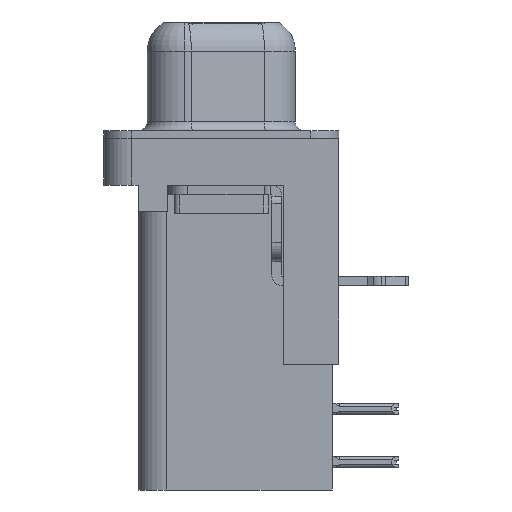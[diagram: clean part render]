
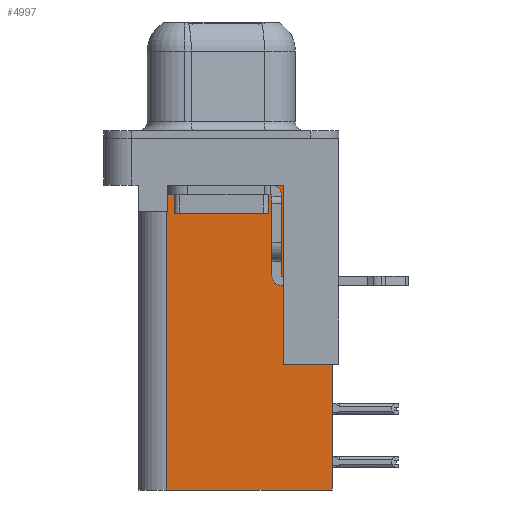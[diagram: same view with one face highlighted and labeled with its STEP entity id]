
A CAD part, left-side view. The second image highlights one B-rep face of the part: STEP entity #4997.
In plain terms, the highlighted planar face has unit normal (-1, 0, 0).
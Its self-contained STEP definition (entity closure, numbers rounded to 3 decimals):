
#1304 = CARTESIAN_POINT ( 'NONE',  ( 3.79, 2.925, -3.9 ) ) ;
#1524 = LINE ( 'NONE', #13325, #19295 ) ;
#1573 = ORIENTED_EDGE ( 'NONE', *, *, #17814, .F. ) ;
#1762 = LINE ( 'NONE', #19416, #5287 ) ;
#1792 = CARTESIAN_POINT ( 'NONE',  ( 3.79, -3.295, -12.05 ) ) ;
#2110 = CARTESIAN_POINT ( 'NONE',  ( 3.79, -3.295, -18.76 ) ) ;
#2253 = DIRECTION ( 'NONE',  ( 0., 0., -1. ) ) ;
#2333 = CARTESIAN_POINT ( 'NONE',  ( 3.79, 2.895, -2.5 ) ) ;
#2478 = CARTESIAN_POINT ( 'NONE',  ( 3.79, 2.925, -18.76 ) ) ;
#2762 = VERTEX_POINT ( 'NONE', #1304 ) ;
#3011 = VECTOR ( 'NONE', #16587, 1000. ) ;
#3033 = DIRECTION ( 'NONE',  ( 0., 1., 0. ) ) ;
#3044 = ORIENTED_EDGE ( 'NONE', *, *, #13088, .T. ) ;
#4007 = CARTESIAN_POINT ( 'NONE',  ( 3.79, 2.925, -18.76 ) ) ;
#4114 = ORIENTED_EDGE ( 'NONE', *, *, #16020, .T. ) ;
#4213 = ORIENTED_EDGE ( 'NONE', *, *, #9682, .F. ) ;
#4594 = CARTESIAN_POINT ( 'NONE',  ( 3.79, -5.925, -2. ) ) ;
#4817 = EDGE_CURVE ( 'NONE', #7934, #2762, #17651, .T. ) ;
#4990 = DIRECTION ( 'NONE',  ( 0., 0., 1. ) ) ;
#4997 = ADVANCED_FACE ( 'NONE', ( #9859 ), #18794, .F. ) ;
#5287 = VECTOR ( 'NONE', #21104, 1000. ) ;
#5357 = CARTESIAN_POINT ( 'NONE',  ( 3.79, -3.295, -18.76 ) ) ;
#5561 = VECTOR ( 'NONE', #8408, 1000. ) ;
#5635 = ORIENTED_EDGE ( 'NONE', *, *, #21165, .T. ) ;
#7562 = EDGE_LOOP ( 'NONE', ( #5635, #3044, #20001, #19280, #1573, #4213, #4114, #18623 ) ) ;
#7934 = VERTEX_POINT ( 'NONE', #2478 ) ;
#8408 = DIRECTION ( 'NONE',  ( 0., 1., 0. ) ) ;
#8547 = VERTEX_POINT ( 'NONE', #11242 ) ;
#9682 = EDGE_CURVE ( 'NONE', #17001, #17704, #16182, .T. ) ;
#9859 = FACE_OUTER_BOUND ( 'NONE', #7562, .T. ) ;
#10117 = CARTESIAN_POINT ( 'NONE',  ( 3.79, 0., -3.9 ) ) ;
#10385 = VECTOR ( 'NONE', #20947, 1000. ) ;
#10558 = CARTESIAN_POINT ( 'NONE',  ( 3.79, -5.925, -18.76 ) ) ;
#10758 = VERTEX_POINT ( 'NONE', #2333 ) ;
#10922 = LINE ( 'NONE', #2110, #10385 ) ;
#11242 = CARTESIAN_POINT ( 'NONE',  ( 3.79, -3.295, -2.5 ) ) ;
#11509 = LINE ( 'NONE', #12554, #20598 ) ;
#12386 = VERTEX_POINT ( 'NONE', #16503 ) ;
#12554 = CARTESIAN_POINT ( 'NONE',  ( 3.79, 2.895, -3.9 ) ) ;
#12839 = AXIS2_PLACEMENT_3D ( 'NONE', #5357, #17766, #17735 ) ;
#13088 = EDGE_CURVE ( 'NONE', #10758, #12386, #11509, .T. ) ;
#13325 = CARTESIAN_POINT ( 'NONE',  ( 3.79, -6.295, -12.05 ) ) ;
#14022 = EDGE_CURVE ( 'NONE', #12386, #2762, #19263, .T. ) ;
#14694 = DIRECTION ( 'NONE',  ( 0., 1., 0. ) ) ;
#15345 = VECTOR ( 'NONE', #14694, 1000. ) ;
#16020 = EDGE_CURVE ( 'NONE', #17001, #22172, #1524, .T. ) ;
#16182 = LINE ( 'NONE', #4594, #3011 ) ;
#16503 = CARTESIAN_POINT ( 'NONE',  ( 3.79, 2.895, -3.9 ) ) ;
#16587 = DIRECTION ( 'NONE',  ( 0., 0., -1. ) ) ;
#17001 = VERTEX_POINT ( 'NONE', #18550 ) ;
#17651 = LINE ( 'NONE', #4007, #21640 ) ;
#17704 = VERTEX_POINT ( 'NONE', #10558 ) ;
#17735 = DIRECTION ( 'NONE',  ( 0., 1., 0. ) ) ;
#17766 = DIRECTION ( 'NONE',  ( 1., 0., 0. ) ) ;
#17781 = EDGE_CURVE ( 'NONE', #22172, #8547, #10922, .T. ) ;
#17814 = EDGE_CURVE ( 'NONE', #17704, #7934, #1762, .T. ) ;
#18550 = CARTESIAN_POINT ( 'NONE',  ( 3.79, -5.925, -12.05 ) ) ;
#18623 = ORIENTED_EDGE ( 'NONE', *, *, #17781, .T. ) ;
#18794 = PLANE ( 'NONE',  #12839 ) ;
#19263 = LINE ( 'NONE', #10117, #5561 ) ;
#19280 = ORIENTED_EDGE ( 'NONE', *, *, #4817, .F. ) ;
#19295 = VECTOR ( 'NONE', #3033, 1000. ) ;
#19416 = CARTESIAN_POINT ( 'NONE',  ( 3.79, -3.295, -18.76 ) ) ;
#19943 = LINE ( 'NONE', #21497, #15345 ) ;
#20001 = ORIENTED_EDGE ( 'NONE', *, *, #14022, .T. ) ;
#20598 = VECTOR ( 'NONE', #2253, 1000. ) ;
#20947 = DIRECTION ( 'NONE',  ( 0., 0., 1. ) ) ;
#21104 = DIRECTION ( 'NONE',  ( 0., 1., 0. ) ) ;
#21165 = EDGE_CURVE ( 'NONE', #8547, #10758, #19943, .T. ) ;
#21497 = CARTESIAN_POINT ( 'NONE',  ( 3.79, -3.295, -2.5 ) ) ;
#21640 = VECTOR ( 'NONE', #4990, 1000. ) ;
#22172 = VERTEX_POINT ( 'NONE', #1792 ) ;
